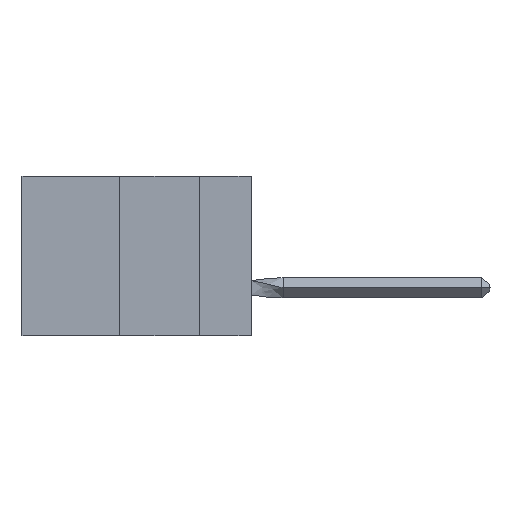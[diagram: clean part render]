
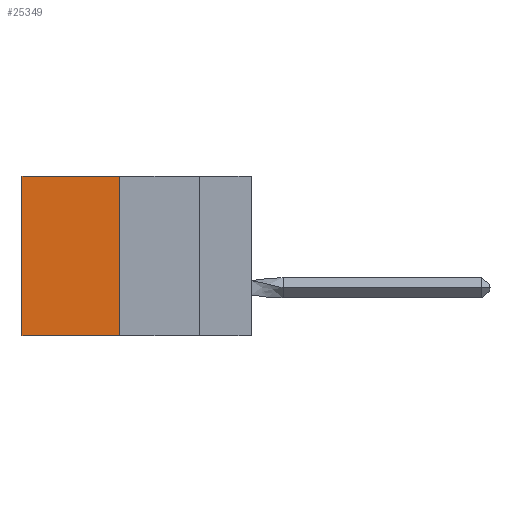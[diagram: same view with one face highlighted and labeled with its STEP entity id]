
A CAD part, left-side view. The second image highlights one B-rep face of the part: STEP entity #25349.
In plain terms, the highlighted planar face has unit normal (-1, 0, 0).
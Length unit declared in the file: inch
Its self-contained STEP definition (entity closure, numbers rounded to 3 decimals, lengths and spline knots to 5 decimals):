
#497 = DIRECTION ( 'NONE',  ( 0., 0., -1. ) ) ;
#1041 = VERTEX_POINT ( 'NONE', #27869 ) ;
#3294 = EDGE_CURVE ( 'NONE', #24367, #1041, #6990, .T. ) ;
#3688 = CARTESIAN_POINT ( 'NONE',  ( 0.305, 0.72, -0.5 ) ) ;
#6990 = LINE ( 'NONE', #18358, #12201 ) ;
#7928 = CARTESIAN_POINT ( 'NONE',  ( 0.305, 0.413, -0.5 ) ) ;
#8609 = VERTEX_POINT ( 'NONE', #29238 ) ;
#8629 = DIRECTION ( 'NONE',  ( 0., 0., -1. ) ) ;
#9523 = EDGE_CURVE ( 'NONE', #24367, #8609, #26037, .T. ) ;
#9723 = VERTEX_POINT ( 'NONE', #41415 ) ;
#12201 = VECTOR ( 'NONE', #29693, 39.37008 ) ;
#12207 = EDGE_CURVE ( 'NONE', #8609, #9723, #35702, .T. ) ;
#12882 = AXIS2_PLACEMENT_3D ( 'NONE', #7928, #42080, #8629 ) ;
#13051 = CARTESIAN_POINT ( 'NONE',  ( 0.305, 0.413, -0.5 ) ) ;
#13587 = FACE_OUTER_BOUND ( 'NONE', #38794, .T. ) ;
#18358 = CARTESIAN_POINT ( 'NONE',  ( 0.305, 0.413, 0. ) ) ;
#19463 = ORIENTED_EDGE ( 'NONE', *, *, #9523, .F. ) ;
#20003 = DIRECTION ( 'NONE',  ( 0., 0., -1. ) ) ;
#20902 = DIRECTION ( 'NONE',  ( 0., 1., 0. ) ) ;
#22298 = ORIENTED_EDGE ( 'NONE', *, *, #41675, .T. ) ;
#24100 = VECTOR ( 'NONE', #497, 39.37008 ) ;
#24367 = VERTEX_POINT ( 'NONE', #31226 ) ;
#25349 = ADVANCED_FACE ( 'NONE', ( #13587 ), #37615, .F. ) ;
#26037 = LINE ( 'NONE', #13051, #35381 ) ;
#26113 = LINE ( 'NONE', #3688, #24100 ) ;
#26868 = VECTOR ( 'NONE', #20902, 39.37008 ) ;
#27869 = CARTESIAN_POINT ( 'NONE',  ( 0.305, 0.72, 0. ) ) ;
#29238 = CARTESIAN_POINT ( 'NONE',  ( 0.305, 0.413, -0.5 ) ) ;
#29693 = DIRECTION ( 'NONE',  ( 0., 1., 0. ) ) ;
#31226 = CARTESIAN_POINT ( 'NONE',  ( 0.305, 0.413, 0. ) ) ;
#35381 = VECTOR ( 'NONE', #20003, 39.37008 ) ;
#35702 = LINE ( 'NONE', #36974, #26868 ) ;
#36549 = ORIENTED_EDGE ( 'NONE', *, *, #12207, .F. ) ;
#36974 = CARTESIAN_POINT ( 'NONE',  ( 0.305, 0.413, -0.5 ) ) ;
#37615 = PLANE ( 'NONE',  #12882 ) ;
#38794 = EDGE_LOOP ( 'NONE', ( #22298, #36549, #19463, #42633 ) ) ;
#41415 = CARTESIAN_POINT ( 'NONE',  ( 0.305, 0.72, -0.5 ) ) ;
#41675 = EDGE_CURVE ( 'NONE', #1041, #9723, #26113, .T. ) ;
#42080 = DIRECTION ( 'NONE',  ( 1., 0., 0. ) ) ;
#42633 = ORIENTED_EDGE ( 'NONE', *, *, #3294, .T. ) ;
